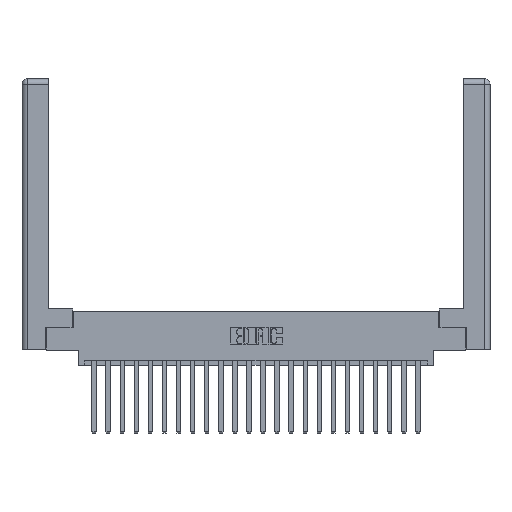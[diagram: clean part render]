
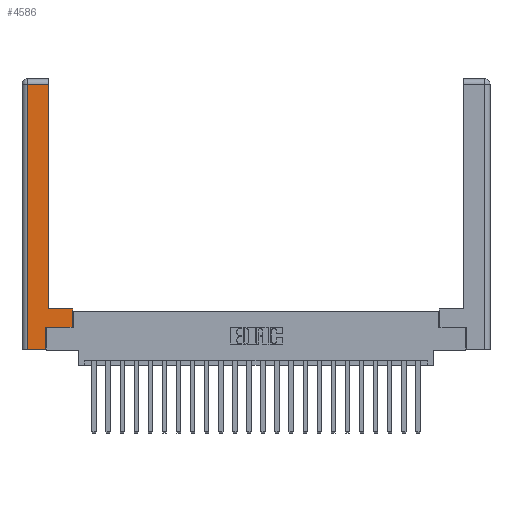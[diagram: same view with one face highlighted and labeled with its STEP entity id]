
A CAD part, top view. The second image highlights one B-rep face of the part: STEP entity #4586.
In plain terms, the highlighted planar face has unit normal (0, 0, 1).
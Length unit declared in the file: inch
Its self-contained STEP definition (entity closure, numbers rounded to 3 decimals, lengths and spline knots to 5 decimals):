
#1174 = CARTESIAN_POINT ( 'NONE',  ( 0.0615, 2.94, 0. ) ) ;
#1467 = DIRECTION ( 'NONE',  ( 0., 0., -1. ) ) ;
#1499 = VERTEX_POINT ( 'NONE', #11951 ) ;
#1702 = DIRECTION ( 'NONE',  ( -1., 0., 0. ) ) ;
#1867 = VERTEX_POINT ( 'NONE', #17393 ) ;
#2009 = CARTESIAN_POINT ( 'NONE',  ( 0.295, 0.45, 0. ) ) ;
#3003 = DIRECTION ( 'NONE',  ( -1., 0., 0. ) ) ;
#3448 = CARTESIAN_POINT ( 'NONE',  ( 0., 0., 0. ) ) ;
#3487 = VECTOR ( 'NONE', #20650, 39.37008 ) ;
#3750 = EDGE_CURVE ( 'NONE', #14940, #21573, #22881, .T. ) ;
#3926 = EDGE_CURVE ( 'NONE', #21573, #17632, #17476, .T. ) ;
#4241 = LINE ( 'NONE', #8987, #14478 ) ;
#4586 = ADVANCED_FACE ( 'NONE', ( #12903 ), #14477, .F. ) ;
#5256 = VERTEX_POINT ( 'NONE', #20337 ) ;
#6016 = CARTESIAN_POINT ( 'NONE',  ( 0.295, 3., 0. ) ) ;
#6021 = CARTESIAN_POINT ( 'NONE',  ( 0.295, 0.45, 0. ) ) ;
#6072 = LINE ( 'NONE', #1174, #17713 ) ;
#6099 = CARTESIAN_POINT ( 'NONE',  ( 0.565, 0.245, 0. ) ) ;
#7306 = LINE ( 'NONE', #22329, #13581 ) ;
#7775 = DIRECTION ( 'NONE',  ( 0., 1., 0. ) ) ;
#8290 = LINE ( 'NONE', #6099, #3487 ) ;
#8308 = ORIENTED_EDGE ( 'NONE', *, *, #13281, .T. ) ;
#8469 = AXIS2_PLACEMENT_3D ( 'NONE', #3448, #1467, #1702 ) ;
#8987 = CARTESIAN_POINT ( 'NONE',  ( 0.0615, 0., 0. ) ) ;
#9508 = CARTESIAN_POINT ( 'NONE',  ( 0.295, 2.94, 0. ) ) ;
#10948 = DIRECTION ( 'NONE',  ( -1., 0., 0. ) ) ;
#11014 = CARTESIAN_POINT ( 'NONE',  ( 0.0615, 2.94, 0. ) ) ;
#11178 = VERTEX_POINT ( 'NONE', #11014 ) ;
#11324 = ORIENTED_EDGE ( 'NONE', *, *, #20144, .T. ) ;
#11547 = EDGE_CURVE ( 'NONE', #17632, #11178, #6072, .T. ) ;
#11919 = CARTESIAN_POINT ( 'NONE',  ( 0.565, 0.45, 0. ) ) ;
#11951 = CARTESIAN_POINT ( 'NONE',  ( 0.565, 0.245, 0. ) ) ;
#12528 = CARTESIAN_POINT ( 'NONE',  ( 0.565, 0.45, 0. ) ) ;
#12903 = FACE_OUTER_BOUND ( 'NONE', #16113, .T. ) ;
#13281 = EDGE_CURVE ( 'NONE', #1867, #5256, #7306, .T. ) ;
#13581 = VECTOR ( 'NONE', #19079, 39.37008 ) ;
#13921 = LINE ( 'NONE', #11919, #19917 ) ;
#14477 = PLANE ( 'NONE',  #8469 ) ;
#14478 = VECTOR ( 'NONE', #18206, 39.37008 ) ;
#14660 = ORIENTED_EDGE ( 'NONE', *, *, #11547, .T. ) ;
#14940 = VERTEX_POINT ( 'NONE', #12528 ) ;
#14978 = LINE ( 'NONE', #20887, #22920 ) ;
#15154 = ORIENTED_EDGE ( 'NONE', *, *, #22908, .T. ) ;
#15799 = ORIENTED_EDGE ( 'NONE', *, *, #17854, .T. ) ;
#16113 = EDGE_LOOP ( 'NONE', ( #19938, #14660, #15799, #11324, #8308, #15154, #22493, #18925 ) ) ;
#17221 = EDGE_CURVE ( 'NONE', #1499, #14940, #13921, .T. ) ;
#17393 = CARTESIAN_POINT ( 'NONE',  ( 0.265, 0., 0. ) ) ;
#17476 = LINE ( 'NONE', #6016, #20351 ) ;
#17632 = VERTEX_POINT ( 'NONE', #9508 ) ;
#17713 = VECTOR ( 'NONE', #3003, 39.37008 ) ;
#17854 = EDGE_CURVE ( 'NONE', #11178, #19109, #4241, .T. ) ;
#18206 = DIRECTION ( 'NONE',  ( 0., -1., 0. ) ) ;
#18925 = ORIENTED_EDGE ( 'NONE', *, *, #3750, .T. ) ;
#18935 = VECTOR ( 'NONE', #10948, 39.37008 ) ;
#19079 = DIRECTION ( 'NONE',  ( 0., 1., 0. ) ) ;
#19109 = VERTEX_POINT ( 'NONE', #22027 ) ;
#19917 = VECTOR ( 'NONE', #23023, 39.37008 ) ;
#19938 = ORIENTED_EDGE ( 'NONE', *, *, #3926, .T. ) ;
#20144 = EDGE_CURVE ( 'NONE', #19109, #1867, #14978, .T. ) ;
#20337 = CARTESIAN_POINT ( 'NONE',  ( 0.265, 0.245, 0. ) ) ;
#20351 = VECTOR ( 'NONE', #7775, 39.37008 ) ;
#20650 = DIRECTION ( 'NONE',  ( 1., 0., 0. ) ) ;
#20887 = CARTESIAN_POINT ( 'NONE',  ( 0.265, 0., 0. ) ) ;
#21573 = VERTEX_POINT ( 'NONE', #6021 ) ;
#22027 = CARTESIAN_POINT ( 'NONE',  ( 0.0615, 0., 0. ) ) ;
#22329 = CARTESIAN_POINT ( 'NONE',  ( 0.265, 0.245, 0. ) ) ;
#22493 = ORIENTED_EDGE ( 'NONE', *, *, #17221, .T. ) ;
#22850 = DIRECTION ( 'NONE',  ( 1., 0., 0. ) ) ;
#22881 = LINE ( 'NONE', #2009, #18935 ) ;
#22908 = EDGE_CURVE ( 'NONE', #5256, #1499, #8290, .T. ) ;
#22920 = VECTOR ( 'NONE', #22850, 39.37008 ) ;
#23023 = DIRECTION ( 'NONE',  ( 0., 1., 0. ) ) ;
